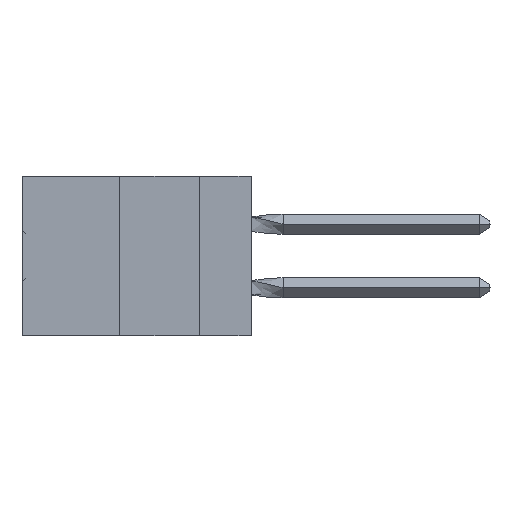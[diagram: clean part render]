
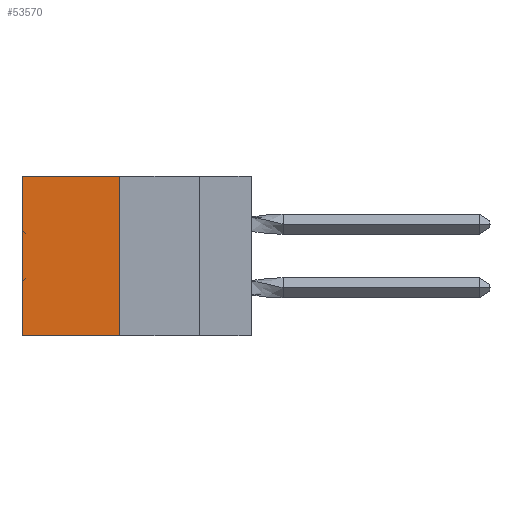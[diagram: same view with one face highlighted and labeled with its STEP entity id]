
A CAD part, left-side view. The second image highlights one B-rep face of the part: STEP entity #53570.
In plain terms, the highlighted planar face has unit normal (-1, 0, 0).
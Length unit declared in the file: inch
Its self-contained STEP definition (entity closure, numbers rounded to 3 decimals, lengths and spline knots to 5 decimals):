
#2699 = CARTESIAN_POINT ( 'NONE',  ( 0.305, 0.413, -0.5 ) ) ;
#3135 = ORIENTED_EDGE ( 'NONE', *, *, #34049, .T. ) ;
#5810 = VECTOR ( 'NONE', #44164, 39.37008 ) ;
#7576 = DIRECTION ( 'NONE',  ( 0., 1., 0. ) ) ;
#8594 = EDGE_CURVE ( 'NONE', #19181, #44524, #17329, .T. ) ;
#9129 = EDGE_CURVE ( 'NONE', #12397, #33422, #33854, .T. ) ;
#9942 = PLANE ( 'NONE',  #10055 ) ;
#10055 = AXIS2_PLACEMENT_3D ( 'NONE', #42147, #46787, #19151 ) ;
#10580 = ORIENTED_EDGE ( 'NONE', *, *, #41217, .F. ) ;
#12397 = VERTEX_POINT ( 'NONE', #50918 ) ;
#14702 = CARTESIAN_POINT ( 'NONE',  ( 0.305, 0.72, -0.5 ) ) ;
#16912 = CARTESIAN_POINT ( 'NONE',  ( 0.305, 0.72, -0.5 ) ) ;
#17329 = LINE ( 'NONE', #14702, #35372 ) ;
#18287 = CARTESIAN_POINT ( 'NONE',  ( 0.305, 0.413, 0. ) ) ;
#18488 = DIRECTION ( 'NONE',  ( 0., 1., 0. ) ) ;
#18725 = DIRECTION ( 'NONE',  ( 0., 0., -1. ) ) ;
#19151 = DIRECTION ( 'NONE',  ( 0., 0., -1. ) ) ;
#19181 = VERTEX_POINT ( 'NONE', #40638 ) ;
#22144 = FACE_OUTER_BOUND ( 'NONE', #38613, .T. ) ;
#22188 = LINE ( 'NONE', #18287, #57555 ) ;
#24762 = VECTOR ( 'NONE', #7576, 39.37008 ) ;
#33422 = VERTEX_POINT ( 'NONE', #40154 ) ;
#33854 = LINE ( 'NONE', #2699, #5810 ) ;
#34049 = EDGE_CURVE ( 'NONE', #12397, #19181, #22188, .T. ) ;
#34791 = ORIENTED_EDGE ( 'NONE', *, *, #8594, .T. ) ;
#34938 = CARTESIAN_POINT ( 'NONE',  ( 0.305, 0.413, -0.5 ) ) ;
#35372 = VECTOR ( 'NONE', #18725, 39.37008 ) ;
#38613 = EDGE_LOOP ( 'NONE', ( #34791, #10580, #52295, #3135 ) ) ;
#40154 = CARTESIAN_POINT ( 'NONE',  ( 0.305, 0.413, -0.5 ) ) ;
#40638 = CARTESIAN_POINT ( 'NONE',  ( 0.305, 0.72, 0. ) ) ;
#41217 = EDGE_CURVE ( 'NONE', #33422, #44524, #58660, .T. ) ;
#42147 = CARTESIAN_POINT ( 'NONE',  ( 0.305, 0.413, -0.5 ) ) ;
#44164 = DIRECTION ( 'NONE',  ( 0., 0., -1. ) ) ;
#44524 = VERTEX_POINT ( 'NONE', #16912 ) ;
#46787 = DIRECTION ( 'NONE',  ( 1., 0., 0. ) ) ;
#50918 = CARTESIAN_POINT ( 'NONE',  ( 0.305, 0.413, 0. ) ) ;
#52295 = ORIENTED_EDGE ( 'NONE', *, *, #9129, .F. ) ;
#53570 = ADVANCED_FACE ( 'NONE', ( #22144 ), #9942, .F. ) ;
#57555 = VECTOR ( 'NONE', #18488, 39.37008 ) ;
#58660 = LINE ( 'NONE', #34938, #24762 ) ;
